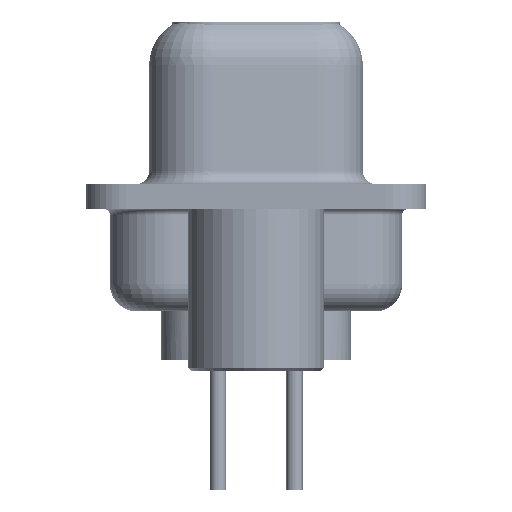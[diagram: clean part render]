
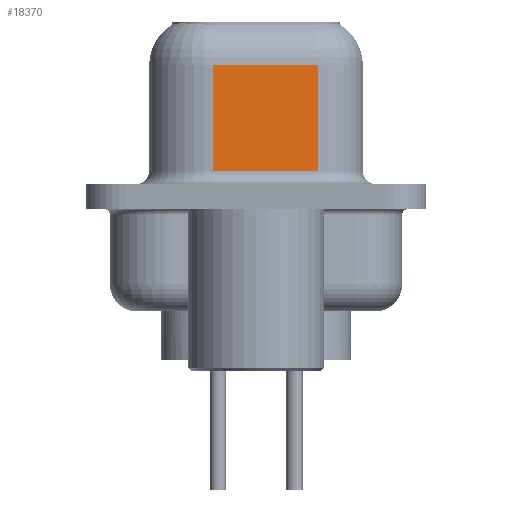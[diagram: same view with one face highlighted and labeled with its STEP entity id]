
A CAD part, left-side view. The second image highlights one B-rep face of the part: STEP entity #18370.
In plain terms, the highlighted planar face has unit normal (-0.985, -0.174, 0).
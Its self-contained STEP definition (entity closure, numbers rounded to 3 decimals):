
#829 = EDGE_CURVE ( 'NONE', #25016, #9152, #5079, .T. ) ;
#879 = DIRECTION ( 'NONE',  ( 0.985, 0.174, 0. ) ) ;
#1111 = ORIENTED_EDGE ( 'NONE', *, *, #26196, .F. ) ;
#2882 = CARTESIAN_POINT ( 'NONE',  ( 5.038, -2.297, 4.85 ) ) ;
#3463 = VECTOR ( 'NONE', #15571, 1000. ) ;
#3572 = AXIS2_PLACEMENT_3D ( 'NONE', #20587, #879, #23048 ) ;
#3765 = CARTESIAN_POINT ( 'NONE',  ( 5.038, -2.297, 6.6 ) ) ;
#4122 = VECTOR ( 'NONE', #22586, 1000. ) ;
#4920 = ORIENTED_EDGE ( 'NONE', *, *, #13769, .T. ) ;
#5079 = LINE ( 'NONE', #2882, #4122 ) ;
#6660 = VECTOR ( 'NONE', #13025, 1000. ) ;
#6766 = CARTESIAN_POINT ( 'NONE',  ( 4.35, 1.603, 6.6 ) ) ;
#7053 = CARTESIAN_POINT ( 'NONE',  ( 4.35, 1.603, 4.85 ) ) ;
#7843 = VECTOR ( 'NONE', #16251, 1000. ) ;
#8695 = EDGE_CURVE ( 'NONE', #9152, #15011, #9493, .T. ) ;
#9152 = VERTEX_POINT ( 'NONE', #7053 ) ;
#9493 = LINE ( 'NONE', #6766, #3463 ) ;
#9753 = LINE ( 'NONE', #18994, #7843 ) ;
#9916 = ORIENTED_EDGE ( 'NONE', *, *, #8695, .T. ) ;
#13025 = DIRECTION ( 'NONE',  ( 0., 0., -1. ) ) ;
#13769 = EDGE_CURVE ( 'NONE', #15011, #25779, #9753, .T. ) ;
#14885 = CARTESIAN_POINT ( 'NONE',  ( 4.35, 1.603, 0.95 ) ) ;
#15011 = VERTEX_POINT ( 'NONE', #14885 ) ;
#15571 = DIRECTION ( 'NONE',  ( 0., 0., -1. ) ) ;
#16251 = DIRECTION ( 'NONE',  ( 0.174, -0.985, 0. ) ) ;
#17096 = LINE ( 'NONE', #3765, #6660 ) ;
#18370 = ADVANCED_FACE ( 'NONE', ( #20734 ), #22608, .F. ) ;
#18625 = EDGE_LOOP ( 'NONE', ( #1111, #28199, #9916, #4920 ) ) ;
#18994 = CARTESIAN_POINT ( 'NONE',  ( 5.038, -2.297, 0.95 ) ) ;
#20587 = CARTESIAN_POINT ( 'NONE',  ( 5.038, -2.297, 6.6 ) ) ;
#20734 = FACE_OUTER_BOUND ( 'NONE', #18625, .T. ) ;
#22586 = DIRECTION ( 'NONE',  ( -0.174, 0.985, 0. ) ) ;
#22608 = PLANE ( 'NONE',  #3572 ) ;
#23048 = DIRECTION ( 'NONE',  ( -0.174, 0.985, 0. ) ) ;
#25016 = VERTEX_POINT ( 'NONE', #28349 ) ;
#25779 = VERTEX_POINT ( 'NONE', #28275 ) ;
#26196 = EDGE_CURVE ( 'NONE', #25016, #25779, #17096, .T. ) ;
#28199 = ORIENTED_EDGE ( 'NONE', *, *, #829, .T. ) ;
#28275 = CARTESIAN_POINT ( 'NONE',  ( 5.038, -2.297, 0.95 ) ) ;
#28349 = CARTESIAN_POINT ( 'NONE',  ( 5.038, -2.297, 4.85 ) ) ;
